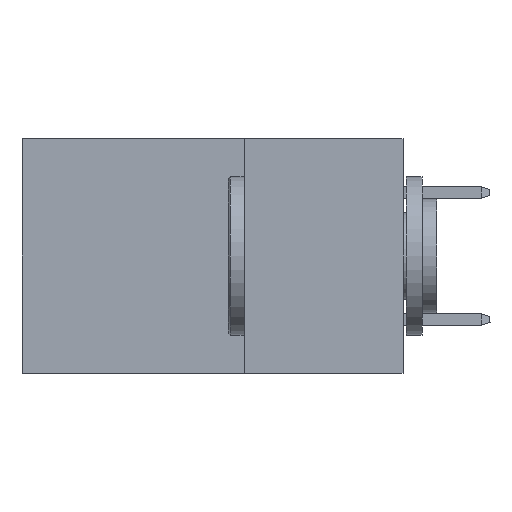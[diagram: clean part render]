
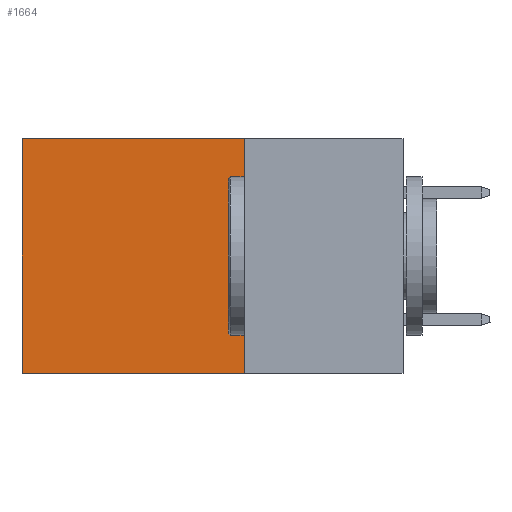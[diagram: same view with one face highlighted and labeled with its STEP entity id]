
A CAD part, left-side view. The second image highlights one B-rep face of the part: STEP entity #1664.
In plain terms, the highlighted planar face has unit normal (-1, 0, 0).
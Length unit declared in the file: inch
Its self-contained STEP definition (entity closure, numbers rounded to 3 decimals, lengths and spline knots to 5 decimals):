
#1664 = ADVANCED_FACE ( 'NONE', ( #12101 ), #19741, .F. ) ;
#1856 = LINE ( 'NONE', #21639, #4529 ) ;
#2260 = CARTESIAN_POINT ( 'NONE',  ( 0.2875, 0.25, 0. ) ) ;
#2382 = EDGE_LOOP ( 'NONE', ( #24784, #21645, #18169, #16069 ) ) ;
#2418 = VERTEX_POINT ( 'NONE', #18932 ) ;
#2433 = CARTESIAN_POINT ( 'NONE',  ( 0.2875, 0.25, -0.37 ) ) ;
#2948 = VERTEX_POINT ( 'NONE', #3941 ) ;
#3424 = EDGE_CURVE ( 'NONE', #2418, #2948, #17768, .T. ) ;
#3941 = CARTESIAN_POINT ( 'NONE',  ( 0.2875, 0.6, 0. ) ) ;
#4401 = VECTOR ( 'NONE', #15899, 39.37008 ) ;
#4529 = VECTOR ( 'NONE', #19339, 39.37008 ) ;
#6253 = EDGE_CURVE ( 'NONE', #24054, #25104, #14234, .T. ) ;
#6718 = VECTOR ( 'NONE', #13574, 39.37008 ) ;
#7341 = EDGE_CURVE ( 'NONE', #2418, #24054, #17091, .T. ) ;
#8111 = CARTESIAN_POINT ( 'NONE',  ( 0.2875, 0.25, -0.37 ) ) ;
#10066 = DIRECTION ( 'NONE',  ( 1., 0., 0. ) ) ;
#11535 = CARTESIAN_POINT ( 'NONE',  ( 0.2875, 0.25, 0. ) ) ;
#12101 = FACE_OUTER_BOUND ( 'NONE', #2382, .T. ) ;
#12222 = DIRECTION ( 'NONE',  ( 0., 0., -1. ) ) ;
#12358 = EDGE_CURVE ( 'NONE', #2948, #25104, #1856, .T. ) ;
#13574 = DIRECTION ( 'NONE',  ( 0., 1., 0. ) ) ;
#14234 = LINE ( 'NONE', #8111, #4401 ) ;
#15899 = DIRECTION ( 'NONE',  ( 0., 1., 0. ) ) ;
#16069 = ORIENTED_EDGE ( 'NONE', *, *, #3424, .T. ) ;
#17091 = LINE ( 'NONE', #18749, #22345 ) ;
#17768 = LINE ( 'NONE', #11535, #6718 ) ;
#18169 = ORIENTED_EDGE ( 'NONE', *, *, #7341, .F. ) ;
#18632 = DIRECTION ( 'NONE',  ( 0., 0., -1. ) ) ;
#18749 = CARTESIAN_POINT ( 'NONE',  ( 0.2875, 0.25, 0. ) ) ;
#18932 = CARTESIAN_POINT ( 'NONE',  ( 0.2875, 0.25, 0. ) ) ;
#19329 = CARTESIAN_POINT ( 'NONE',  ( 0.2875, 0.6, -0.37 ) ) ;
#19339 = DIRECTION ( 'NONE',  ( 0., 0., -1. ) ) ;
#19741 = PLANE ( 'NONE',  #24052 ) ;
#21639 = CARTESIAN_POINT ( 'NONE',  ( 0.2875, 0.6, 0. ) ) ;
#21645 = ORIENTED_EDGE ( 'NONE', *, *, #6253, .F. ) ;
#22345 = VECTOR ( 'NONE', #18632, 39.37008 ) ;
#24052 = AXIS2_PLACEMENT_3D ( 'NONE', #2260, #10066, #12222 ) ;
#24054 = VERTEX_POINT ( 'NONE', #2433 ) ;
#24784 = ORIENTED_EDGE ( 'NONE', *, *, #12358, .T. ) ;
#25104 = VERTEX_POINT ( 'NONE', #19329 ) ;
